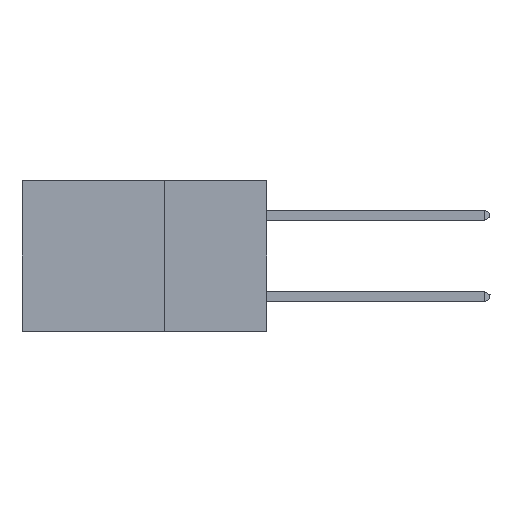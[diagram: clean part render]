
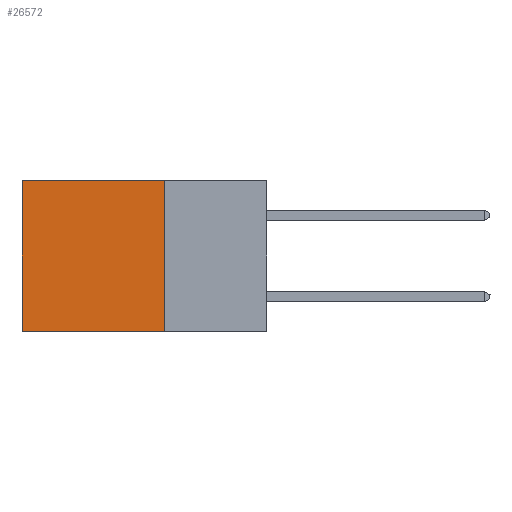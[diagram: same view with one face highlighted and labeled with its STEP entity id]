
A CAD part, left-side view. The second image highlights one B-rep face of the part: STEP entity #26572.
In plain terms, the highlighted planar face has unit normal (-1, 0, 0).
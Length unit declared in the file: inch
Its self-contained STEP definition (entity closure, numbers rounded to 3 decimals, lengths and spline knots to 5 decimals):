
#1189 = EDGE_CURVE ( 'NONE', #24531, #13861, #3468, .T. ) ;
#2211 = EDGE_CURVE ( 'NONE', #24531, #17683, #35461, .T. ) ;
#3468 = LINE ( 'NONE', #7478, #27503 ) ;
#4749 = LINE ( 'NONE', #22848, #15226 ) ;
#4768 = CARTESIAN_POINT ( 'NONE',  ( 0.2875, 0.25, 0. ) ) ;
#6443 = DIRECTION ( 'NONE',  ( 0., 0., -1. ) ) ;
#7478 = CARTESIAN_POINT ( 'NONE',  ( 0.2875, 0.25, 0. ) ) ;
#8360 = CARTESIAN_POINT ( 'NONE',  ( 0.2875, 0.6, -0.37 ) ) ;
#9052 = LINE ( 'NONE', #30456, #31328 ) ;
#13389 = ORIENTED_EDGE ( 'NONE', *, *, #1189, .T. ) ;
#13861 = VERTEX_POINT ( 'NONE', #20084 ) ;
#14013 = VECTOR ( 'NONE', #18954, 39.37008 ) ;
#15058 = ORIENTED_EDGE ( 'NONE', *, *, #17291, .T. ) ;
#15226 = VECTOR ( 'NONE', #6443, 39.37008 ) ;
#16388 = CARTESIAN_POINT ( 'NONE',  ( 0.2875, 0.25, -0.37 ) ) ;
#16420 = DIRECTION ( 'NONE',  ( 0., 1., 0. ) ) ;
#16793 = DIRECTION ( 'NONE',  ( 0., 0., -1. ) ) ;
#17032 = DIRECTION ( 'NONE',  ( 1., 0., 0. ) ) ;
#17291 = EDGE_CURVE ( 'NONE', #13861, #20261, #4749, .T. ) ;
#17683 = VERTEX_POINT ( 'NONE', #16388 ) ;
#18954 = DIRECTION ( 'NONE',  ( 0., 0., -1. ) ) ;
#19847 = CARTESIAN_POINT ( 'NONE',  ( 0.2875, 0.25, 0. ) ) ;
#20084 = CARTESIAN_POINT ( 'NONE',  ( 0.2875, 0.6, 0. ) ) ;
#20261 = VERTEX_POINT ( 'NONE', #8360 ) ;
#21648 = DIRECTION ( 'NONE',  ( 0., 1., 0. ) ) ;
#21949 = ORIENTED_EDGE ( 'NONE', *, *, #2211, .F. ) ;
#22848 = CARTESIAN_POINT ( 'NONE',  ( 0.2875, 0.6, 0. ) ) ;
#22978 = AXIS2_PLACEMENT_3D ( 'NONE', #36119, #17032, #16793 ) ;
#24531 = VERTEX_POINT ( 'NONE', #19847 ) ;
#25849 = FACE_OUTER_BOUND ( 'NONE', #28893, .T. ) ;
#26572 = ADVANCED_FACE ( 'NONE', ( #25849 ), #33785, .F. ) ;
#27503 = VECTOR ( 'NONE', #21648, 39.37008 ) ;
#28139 = ORIENTED_EDGE ( 'NONE', *, *, #32792, .F. ) ;
#28893 = EDGE_LOOP ( 'NONE', ( #15058, #28139, #21949, #13389 ) ) ;
#30456 = CARTESIAN_POINT ( 'NONE',  ( 0.2875, 0.25, -0.37 ) ) ;
#31328 = VECTOR ( 'NONE', #16420, 39.37008 ) ;
#32792 = EDGE_CURVE ( 'NONE', #17683, #20261, #9052, .T. ) ;
#33785 = PLANE ( 'NONE',  #22978 ) ;
#35461 = LINE ( 'NONE', #4768, #14013 ) ;
#36119 = CARTESIAN_POINT ( 'NONE',  ( 0.2875, 0.25, 0. ) ) ;
